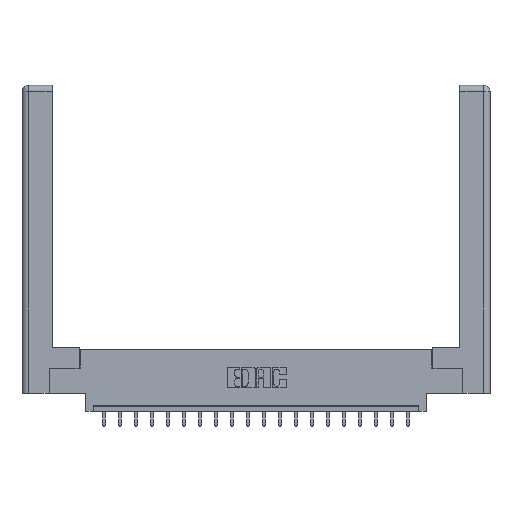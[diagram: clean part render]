
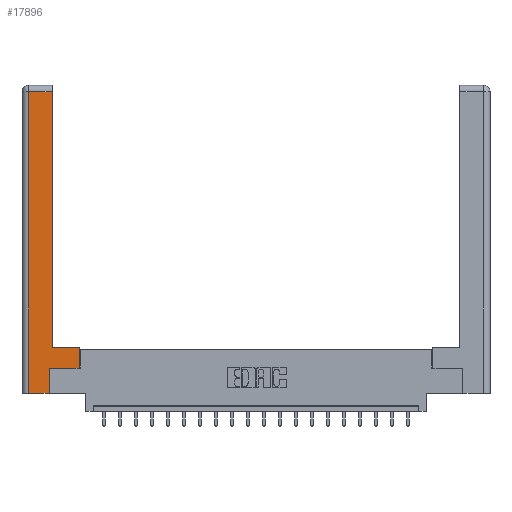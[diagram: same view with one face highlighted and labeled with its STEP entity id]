
A CAD part, top view. The second image highlights one B-rep face of the part: STEP entity #17896.
In plain terms, the highlighted planar face has unit normal (0, 0, 1).
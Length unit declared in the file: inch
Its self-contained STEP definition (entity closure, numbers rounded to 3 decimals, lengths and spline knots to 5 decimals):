
#5 = VERTEX_POINT ( 'NONE', #12808 ) ;
#516 = ORIENTED_EDGE ( 'NONE', *, *, #18825, .T. ) ;
#533 = ORIENTED_EDGE ( 'NONE', *, *, #13170, .T. ) ;
#744 = VERTEX_POINT ( 'NONE', #9169 ) ;
#809 = CARTESIAN_POINT ( 'NONE',  ( 0.565, 0.45, 0. ) ) ;
#904 = CARTESIAN_POINT ( 'NONE',  ( 0.565, 0.45, 0. ) ) ;
#1545 = CARTESIAN_POINT ( 'NONE',  ( 0.265, 0., 0. ) ) ;
#1918 = CARTESIAN_POINT ( 'NONE',  ( 0.295, 0.45, 0. ) ) ;
#2867 = CARTESIAN_POINT ( 'NONE',  ( 0.265, 0.245, 0. ) ) ;
#3077 = VECTOR ( 'NONE', #4184, 39.37008 ) ;
#3221 = VECTOR ( 'NONE', #11003, 39.37008 ) ;
#3235 = FACE_OUTER_BOUND ( 'NONE', #9891, .T. ) ;
#3620 = CARTESIAN_POINT ( 'NONE',  ( 0.565, 0.245, 0. ) ) ;
#3873 = CARTESIAN_POINT ( 'NONE',  ( 0.295, 3., 0. ) ) ;
#4184 = DIRECTION ( 'NONE',  ( 0., 1., 0. ) ) ;
#4201 = ORIENTED_EDGE ( 'NONE', *, *, #6544, .T. ) ;
#4580 = CARTESIAN_POINT ( 'NONE',  ( 0.0615, 2.94, 0. ) ) ;
#4675 = CARTESIAN_POINT ( 'NONE',  ( 0.265, 0.245, 0. ) ) ;
#5198 = LINE ( 'NONE', #7890, #3221 ) ;
#5792 = VECTOR ( 'NONE', #16148, 39.37008 ) ;
#5906 = CARTESIAN_POINT ( 'NONE',  ( 0., 0., 0. ) ) ;
#6544 = EDGE_CURVE ( 'NONE', #5, #17990, #7926, .T. ) ;
#6786 = DIRECTION ( 'NONE',  ( 1., 0., 0. ) ) ;
#7516 = VERTEX_POINT ( 'NONE', #8700 ) ;
#7695 = EDGE_CURVE ( 'NONE', #7516, #5, #18828, .T. ) ;
#7844 = DIRECTION ( 'NONE',  ( 0., 1., 0. ) ) ;
#7890 = CARTESIAN_POINT ( 'NONE',  ( 0.0615, 0., 0. ) ) ;
#7926 = LINE ( 'NONE', #4675, #18841 ) ;
#8700 = CARTESIAN_POINT ( 'NONE',  ( 0.0615, 0., 0. ) ) ;
#8701 = VECTOR ( 'NONE', #6786, 39.37008 ) ;
#8893 = DIRECTION ( 'NONE',  ( -1., 0., 0. ) ) ;
#9169 = CARTESIAN_POINT ( 'NONE',  ( 0.295, 2.94, 0. ) ) ;
#9260 = VERTEX_POINT ( 'NONE', #809 ) ;
#9883 = ORIENTED_EDGE ( 'NONE', *, *, #11887, .T. ) ;
#9891 = EDGE_LOOP ( 'NONE', ( #533, #16332, #516, #13356, #4201, #9883, #10988, #16072 ) ) ;
#10126 = EDGE_CURVE ( 'NONE', #17645, #9260, #18702, .T. ) ;
#10213 = AXIS2_PLACEMENT_3D ( 'NONE', #5906, #15107, #8893 ) ;
#10988 = ORIENTED_EDGE ( 'NONE', *, *, #10126, .T. ) ;
#11003 = DIRECTION ( 'NONE',  ( 0., -1., 0. ) ) ;
#11887 = EDGE_CURVE ( 'NONE', #17990, #17645, #12908, .T. ) ;
#12145 = PLANE ( 'NONE',  #10213 ) ;
#12447 = VERTEX_POINT ( 'NONE', #18415 ) ;
#12535 = DIRECTION ( 'NONE',  ( 1., 0., 0. ) ) ;
#12808 = CARTESIAN_POINT ( 'NONE',  ( 0.265, 0., 0. ) ) ;
#12908 = LINE ( 'NONE', #3620, #8701 ) ;
#13170 = EDGE_CURVE ( 'NONE', #12447, #744, #20081, .T. ) ;
#13254 = DIRECTION ( 'NONE',  ( 0., 1., 0. ) ) ;
#13356 = ORIENTED_EDGE ( 'NONE', *, *, #7695, .T. ) ;
#13445 = CARTESIAN_POINT ( 'NONE',  ( 0.565, 0.245, 0. ) ) ;
#13471 = EDGE_CURVE ( 'NONE', #744, #17682, #13603, .T. ) ;
#13603 = LINE ( 'NONE', #4580, #20310 ) ;
#15107 = DIRECTION ( 'NONE',  ( 0., 0., -1. ) ) ;
#15430 = DIRECTION ( 'NONE',  ( -1., 0., 0. ) ) ;
#15585 = VECTOR ( 'NONE', #12535, 39.37008 ) ;
#15847 = VECTOR ( 'NONE', #13254, 39.37008 ) ;
#16072 = ORIENTED_EDGE ( 'NONE', *, *, #16118, .T. ) ;
#16118 = EDGE_CURVE ( 'NONE', #9260, #12447, #18440, .T. ) ;
#16148 = DIRECTION ( 'NONE',  ( -1., 0., 0. ) ) ;
#16332 = ORIENTED_EDGE ( 'NONE', *, *, #13471, .T. ) ;
#17645 = VERTEX_POINT ( 'NONE', #13445 ) ;
#17682 = VERTEX_POINT ( 'NONE', #19196 ) ;
#17896 = ADVANCED_FACE ( 'NONE', ( #3235 ), #12145, .F. ) ;
#17990 = VERTEX_POINT ( 'NONE', #2867 ) ;
#18415 = CARTESIAN_POINT ( 'NONE',  ( 0.295, 0.45, 0. ) ) ;
#18440 = LINE ( 'NONE', #1918, #5792 ) ;
#18702 = LINE ( 'NONE', #904, #3077 ) ;
#18825 = EDGE_CURVE ( 'NONE', #17682, #7516, #5198, .T. ) ;
#18828 = LINE ( 'NONE', #1545, #15585 ) ;
#18841 = VECTOR ( 'NONE', #7844, 39.37008 ) ;
#19196 = CARTESIAN_POINT ( 'NONE',  ( 0.0615, 2.94, 0. ) ) ;
#20081 = LINE ( 'NONE', #3873, #15847 ) ;
#20310 = VECTOR ( 'NONE', #15430, 39.37008 ) ;
